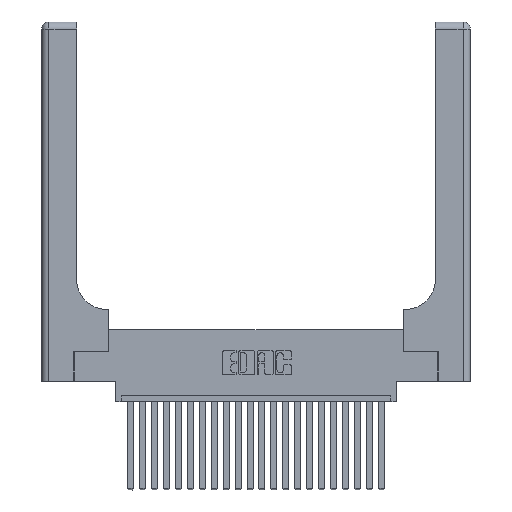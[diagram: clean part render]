
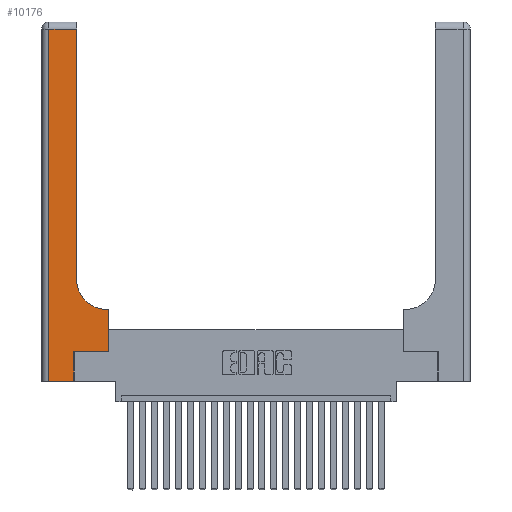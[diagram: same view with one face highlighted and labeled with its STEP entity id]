
A CAD part, top view. The second image highlights one B-rep face of the part: STEP entity #10176.
In plain terms, the highlighted planar face has unit normal (0, 0, 1).
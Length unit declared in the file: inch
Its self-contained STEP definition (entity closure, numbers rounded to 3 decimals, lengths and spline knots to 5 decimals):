
#516 = CARTESIAN_POINT ( 'NONE',  ( 0., 3., 0.37 ) ) ;
#753 = VERTEX_POINT ( 'NONE', #9041 ) ;
#929 = LINE ( 'NONE', #16050, #6196 ) ;
#1232 = DIRECTION ( 'NONE',  ( -1., 0., 0. ) ) ;
#2392 = CARTESIAN_POINT ( 'NONE',  ( 0.5415, 0.6, 0.37 ) ) ;
#2564 = VECTOR ( 'NONE', #5348, 39.37008 ) ;
#3344 = CARTESIAN_POINT ( 'NONE',  ( 0.269, 0.25, 0.37 ) ) ;
#3565 = VECTOR ( 'NONE', #12671, 39.37008 ) ;
#3781 = CARTESIAN_POINT ( 'NONE',  ( 0.269, 0.25, 0.37 ) ) ;
#3927 = CARTESIAN_POINT ( 'NONE',  ( 0.2915, 0.85, 0.37 ) ) ;
#4929 = ORIENTED_EDGE ( 'NONE', *, *, #14875, .T. ) ;
#5097 = ORIENTED_EDGE ( 'NONE', *, *, #11740, .T. ) ;
#5288 = CARTESIAN_POINT ( 'NONE',  ( 0.2915, 0.6, 0.37 ) ) ;
#5348 = DIRECTION ( 'NONE',  ( 0., 1., 0. ) ) ;
#5610 = ORIENTED_EDGE ( 'NONE', *, *, #22247, .T. ) ;
#6196 = VECTOR ( 'NONE', #7948, 39.37008 ) ;
#6353 = VERTEX_POINT ( 'NONE', #15563 ) ;
#6589 = EDGE_CURVE ( 'NONE', #12976, #16460, #929, .T. ) ;
#6684 = VECTOR ( 'NONE', #14664, 39.37008 ) ;
#7063 = CARTESIAN_POINT ( 'NONE',  ( 0.06, 2.94, 0.37 ) ) ;
#7106 = CARTESIAN_POINT ( 'NONE',  ( 0.2915, 3., 0.37 ) ) ;
#7598 = LINE ( 'NONE', #7106, #2564 ) ;
#7785 = CIRCLE ( 'NONE', #11750, 0.25 ) ;
#7808 = LINE ( 'NONE', #3344, #19610 ) ;
#7948 = DIRECTION ( 'NONE',  ( 0., 1., 0. ) ) ;
#8405 = VECTOR ( 'NONE', #9177, 39.37008 ) ;
#8421 = EDGE_CURVE ( 'NONE', #23786, #6353, #7598, .T. ) ;
#8434 = ORIENTED_EDGE ( 'NONE', *, *, #8421, .T. ) ;
#8802 = LINE ( 'NONE', #23777, #18248 ) ;
#9041 = CARTESIAN_POINT ( 'NONE',  ( 0.06, 0., 0.37 ) ) ;
#9177 = DIRECTION ( 'NONE',  ( 0., -1., 0. ) ) ;
#9310 = ORIENTED_EDGE ( 'NONE', *, *, #21305, .T. ) ;
#9434 = ORIENTED_EDGE ( 'NONE', *, *, #12930, .T. ) ;
#10176 = ADVANCED_FACE ( 'NONE', ( #17267 ), #11824, .F. ) ;
#10952 = DIRECTION ( 'NONE',  ( 1., 0., 0. ) ) ;
#11395 = DIRECTION ( 'NONE',  ( 0., 0., -1. ) ) ;
#11740 = EDGE_CURVE ( 'NONE', #753, #12976, #16458, .T. ) ;
#11750 = AXIS2_PLACEMENT_3D ( 'NONE', #17069, #11395, #18960 ) ;
#11824 = PLANE ( 'NONE',  #13760 ) ;
#11858 = CARTESIAN_POINT ( 'NONE',  ( 0.5585, 0.25, 0.37 ) ) ;
#12671 = DIRECTION ( 'NONE',  ( 0., 1., 0. ) ) ;
#12930 = EDGE_CURVE ( 'NONE', #16460, #15921, #7808, .T. ) ;
#12976 = VERTEX_POINT ( 'NONE', #14451 ) ;
#13141 = EDGE_CURVE ( 'NONE', #14906, #753, #13393, .T. ) ;
#13301 = LINE ( 'NONE', #18293, #3565 ) ;
#13393 = LINE ( 'NONE', #22648, #8405 ) ;
#13760 = AXIS2_PLACEMENT_3D ( 'NONE', #516, #21928, #13976 ) ;
#13976 = DIRECTION ( 'NONE',  ( -1., 0., 0. ) ) ;
#14360 = CARTESIAN_POINT ( 'NONE',  ( 0., 0., 0.37 ) ) ;
#14451 = CARTESIAN_POINT ( 'NONE',  ( 0.269, 0., 0.37 ) ) ;
#14664 = DIRECTION ( 'NONE',  ( 1., 0., 0. ) ) ;
#14875 = EDGE_CURVE ( 'NONE', #15921, #17299, #13301, .T. ) ;
#14906 = VERTEX_POINT ( 'NONE', #7063 ) ;
#15563 = CARTESIAN_POINT ( 'NONE',  ( 0.2915, 2.94, 0.37 ) ) ;
#15742 = ORIENTED_EDGE ( 'NONE', *, *, #6589, .T. ) ;
#15919 = VECTOR ( 'NONE', #18499, 39.37008 ) ;
#15921 = VERTEX_POINT ( 'NONE', #11858 ) ;
#16050 = CARTESIAN_POINT ( 'NONE',  ( 0.269, 0., 0.37 ) ) ;
#16458 = LINE ( 'NONE', #14360, #6684 ) ;
#16460 = VERTEX_POINT ( 'NONE', #3781 ) ;
#16509 = VERTEX_POINT ( 'NONE', #2392 ) ;
#17069 = CARTESIAN_POINT ( 'NONE',  ( 0.5415, 0.85, 0.37 ) ) ;
#17267 = FACE_OUTER_BOUND ( 'NONE', #21334, .T. ) ;
#17299 = VERTEX_POINT ( 'NONE', #20093 ) ;
#18248 = VECTOR ( 'NONE', #1232, 39.37008 ) ;
#18289 = LINE ( 'NONE', #5288, #15919 ) ;
#18293 = CARTESIAN_POINT ( 'NONE',  ( 0.5585, 0.25, 0.37 ) ) ;
#18499 = DIRECTION ( 'NONE',  ( -1., 0., 0. ) ) ;
#18960 = DIRECTION ( 'NONE',  ( 1., 0., 0. ) ) ;
#19610 = VECTOR ( 'NONE', #10952, 39.37008 ) ;
#20093 = CARTESIAN_POINT ( 'NONE',  ( 0.5585, 0.6, 0.37 ) ) ;
#20681 = ORIENTED_EDGE ( 'NONE', *, *, #13141, .T. ) ;
#21148 = ORIENTED_EDGE ( 'NONE', *, *, #24342, .T. ) ;
#21305 = EDGE_CURVE ( 'NONE', #17299, #16509, #18289, .T. ) ;
#21334 = EDGE_LOOP ( 'NONE', ( #8434, #5610, #20681, #5097, #15742, #9434, #4929, #9310, #21148 ) ) ;
#21928 = DIRECTION ( 'NONE',  ( 0., 0., -1. ) ) ;
#22247 = EDGE_CURVE ( 'NONE', #6353, #14906, #8802, .T. ) ;
#22648 = CARTESIAN_POINT ( 'NONE',  ( 0.06, 3., 0.37 ) ) ;
#23777 = CARTESIAN_POINT ( 'NONE',  ( 0., 2.94, 0.37 ) ) ;
#23786 = VERTEX_POINT ( 'NONE', #3927 ) ;
#24342 = EDGE_CURVE ( 'NONE', #16509, #23786, #7785, .T. ) ;
